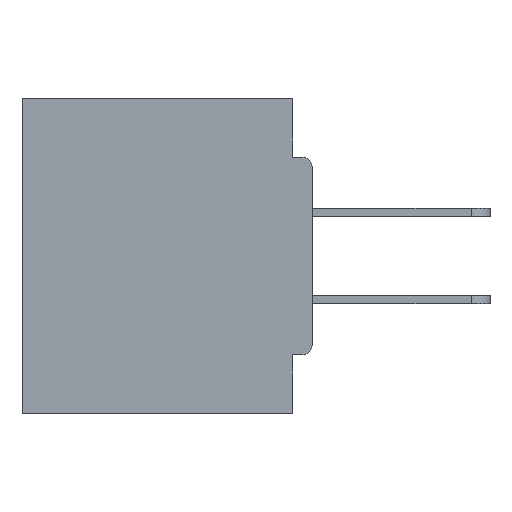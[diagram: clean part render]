
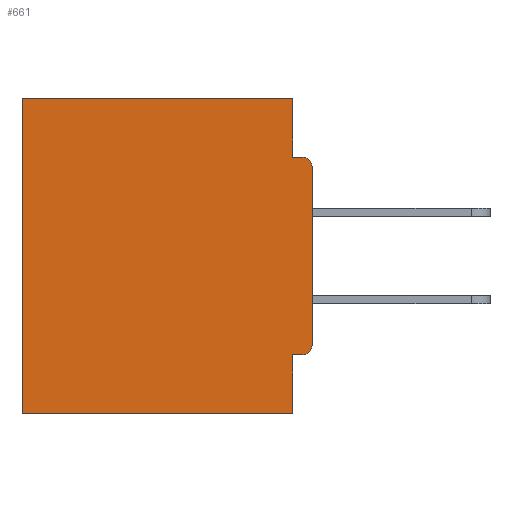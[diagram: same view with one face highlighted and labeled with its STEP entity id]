
A CAD part, left-side view. The second image highlights one B-rep face of the part: STEP entity #661.
In plain terms, the highlighted planar face has unit normal (-1, 0, 0).
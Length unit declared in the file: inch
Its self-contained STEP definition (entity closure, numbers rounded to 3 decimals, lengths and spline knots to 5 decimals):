
#374 = DIRECTION ( 'NONE',  ( 0., 0., -1. ) ) ;
#547 = CARTESIAN_POINT ( 'NONE',  ( 0.298, 0.015, -0.0935 ) ) ;
#661 = ADVANCED_FACE ( 'NONE', ( #4145 ), #21343, .F. ) ;
#782 = CIRCLE ( 'NONE', #31061, 0.015 ) ;
#1140 = AXIS2_PLACEMENT_3D ( 'NONE', #20886, #7166, #15572 ) ;
#1390 = LINE ( 'NONE', #31660, #19876 ) ;
#1512 = LINE ( 'NONE', #6616, #23419 ) ;
#1608 = DIRECTION ( 'NONE',  ( 0., 1., 0. ) ) ;
#1616 = EDGE_CURVE ( 'NONE', #9652, #26575, #33538, .T. ) ;
#1846 = ORIENTED_EDGE ( 'NONE', *, *, #15901, .T. ) ;
#2208 = CARTESIAN_POINT ( 'NONE',  ( 0.298, 0.031, -0.5 ) ) ;
#2293 = VERTEX_POINT ( 'NONE', #23931 ) ;
#2454 = CARTESIAN_POINT ( 'NONE',  ( 0.298, 0., -0.0935 ) ) ;
#2459 = LINE ( 'NONE', #2454, #28231 ) ;
#4145 = FACE_OUTER_BOUND ( 'NONE', #8596, .T. ) ;
#4215 = VERTEX_POINT ( 'NONE', #7844 ) ;
#4438 = CARTESIAN_POINT ( 'NONE',  ( 0.298, 0.46, 0. ) ) ;
#4680 = EDGE_CURVE ( 'NONE', #32366, #9652, #1512, .T. ) ;
#4690 = DIRECTION ( 'NONE',  ( -1., 0., 0. ) ) ;
#4839 = EDGE_CURVE ( 'NONE', #17970, #2293, #15240, .T. ) ;
#5375 = DIRECTION ( 'NONE',  ( 0., 1., 0. ) ) ;
#5784 = VECTOR ( 'NONE', #21494, 39.37008 ) ;
#6072 = ORIENTED_EDGE ( 'NONE', *, *, #30248, .F. ) ;
#6616 = CARTESIAN_POINT ( 'NONE',  ( 0.298, 0.031, -0.5 ) ) ;
#7166 = DIRECTION ( 'NONE',  ( 1., 0., 0. ) ) ;
#7240 = DIRECTION ( 'NONE',  ( 0., 0., -1. ) ) ;
#7844 = CARTESIAN_POINT ( 'NONE',  ( 0.298, 0.015, -0.4065 ) ) ;
#7858 = DIRECTION ( 'NONE',  ( 0., 0., -1. ) ) ;
#8596 = EDGE_LOOP ( 'NONE', ( #32568, #6072, #14424, #16333, #1846, #21913, #14632, #15095, #13992, #29416 ) ) ;
#9015 = VERTEX_POINT ( 'NONE', #30677 ) ;
#9526 = CARTESIAN_POINT ( 'NONE',  ( 0.298, 0., -0.3915 ) ) ;
#9652 = VERTEX_POINT ( 'NONE', #2208 ) ;
#10573 = DIRECTION ( 'NONE',  ( 0., -1., 0. ) ) ;
#11113 = EDGE_CURVE ( 'NONE', #9015, #28204, #24103, .T. ) ;
#12197 = CARTESIAN_POINT ( 'NONE',  ( 0.298, 0.031, 0. ) ) ;
#13992 = ORIENTED_EDGE ( 'NONE', *, *, #20713, .T. ) ;
#14424 = ORIENTED_EDGE ( 'NONE', *, *, #16458, .F. ) ;
#14632 = ORIENTED_EDGE ( 'NONE', *, *, #4680, .F. ) ;
#15095 = ORIENTED_EDGE ( 'NONE', *, *, #24324, .F. ) ;
#15149 = VECTOR ( 'NONE', #1608, 39.37008 ) ;
#15240 = LINE ( 'NONE', #24503, #5784 ) ;
#15329 = DIRECTION ( 'NONE',  ( 0., 0., -1. ) ) ;
#15572 = DIRECTION ( 'NONE',  ( 0., 0., -1. ) ) ;
#15901 = EDGE_CURVE ( 'NONE', #2293, #26575, #29331, .T. ) ;
#16279 = DIRECTION ( 'NONE',  ( -1., 0., 0. ) ) ;
#16333 = ORIENTED_EDGE ( 'NONE', *, *, #4839, .T. ) ;
#16458 = EDGE_CURVE ( 'NONE', #17970, #28552, #1390, .T. ) ;
#16599 = VECTOR ( 'NONE', #374, 39.37008 ) ;
#17931 = CARTESIAN_POINT ( 'NONE',  ( 0.298, 0., -0.4065 ) ) ;
#17970 = VERTEX_POINT ( 'NONE', #12197 ) ;
#19013 = LINE ( 'NONE', #17931, #15149 ) ;
#19853 = CARTESIAN_POINT ( 'NONE',  ( 0.298, 0., 0. ) ) ;
#19876 = VECTOR ( 'NONE', #7240, 39.37008 ) ;
#20713 = EDGE_CURVE ( 'NONE', #4215, #24262, #782, .T. ) ;
#20886 = CARTESIAN_POINT ( 'NONE',  ( 0.298, 0., 0. ) ) ;
#21343 = PLANE ( 'NONE',  #1140 ) ;
#21494 = DIRECTION ( 'NONE',  ( 0., 1., 0. ) ) ;
#21913 = ORIENTED_EDGE ( 'NONE', *, *, #1616, .F. ) ;
#23240 = VECTOR ( 'NONE', #5375, 39.37008 ) ;
#23419 = VECTOR ( 'NONE', #28506, 39.37008 ) ;
#23734 = VECTOR ( 'NONE', #15329, 39.37008 ) ;
#23898 = LINE ( 'NONE', #19853, #16599 ) ;
#23931 = CARTESIAN_POINT ( 'NONE',  ( 0.298, 0.46, 0. ) ) ;
#24103 = CIRCLE ( 'NONE', #33589, 0.015 ) ;
#24262 = VERTEX_POINT ( 'NONE', #9526 ) ;
#24324 = EDGE_CURVE ( 'NONE', #4215, #32366, #19013, .T. ) ;
#24503 = CARTESIAN_POINT ( 'NONE',  ( 0.298, 0., 0. ) ) ;
#26575 = VERTEX_POINT ( 'NONE', #34005 ) ;
#28204 = VERTEX_POINT ( 'NONE', #547 ) ;
#28231 = VECTOR ( 'NONE', #10573, 39.37008 ) ;
#28506 = DIRECTION ( 'NONE',  ( 0., 0., -1. ) ) ;
#28552 = VERTEX_POINT ( 'NONE', #29834 ) ;
#29331 = LINE ( 'NONE', #4438, #23734 ) ;
#29416 = ORIENTED_EDGE ( 'NONE', *, *, #30576, .F. ) ;
#29834 = CARTESIAN_POINT ( 'NONE',  ( 0.298, 0.031, -0.0935 ) ) ;
#30248 = EDGE_CURVE ( 'NONE', #28552, #28204, #2459, .T. ) ;
#30367 = CARTESIAN_POINT ( 'NONE',  ( 0.298, 0.015, -0.1085 ) ) ;
#30576 = EDGE_CURVE ( 'NONE', #9015, #24262, #23898, .T. ) ;
#30677 = CARTESIAN_POINT ( 'NONE',  ( 0.298, 0., -0.1085 ) ) ;
#31061 = AXIS2_PLACEMENT_3D ( 'NONE', #31919, #4690, #32038 ) ;
#31457 = CARTESIAN_POINT ( 'NONE',  ( 0.298, 0.031, -0.4065 ) ) ;
#31660 = CARTESIAN_POINT ( 'NONE',  ( 0.298, 0.031, -0.5 ) ) ;
#31919 = CARTESIAN_POINT ( 'NONE',  ( 0.298, 0.015, -0.3915 ) ) ;
#32038 = DIRECTION ( 'NONE',  ( 0., 0., -1. ) ) ;
#32366 = VERTEX_POINT ( 'NONE', #31457 ) ;
#32568 = ORIENTED_EDGE ( 'NONE', *, *, #11113, .T. ) ;
#33538 = LINE ( 'NONE', #35533, #23240 ) ;
#33589 = AXIS2_PLACEMENT_3D ( 'NONE', #30367, #16279, #7858 ) ;
#34005 = CARTESIAN_POINT ( 'NONE',  ( 0.298, 0.46, -0.5 ) ) ;
#35533 = CARTESIAN_POINT ( 'NONE',  ( 0.298, 0., -0.5 ) ) ;
